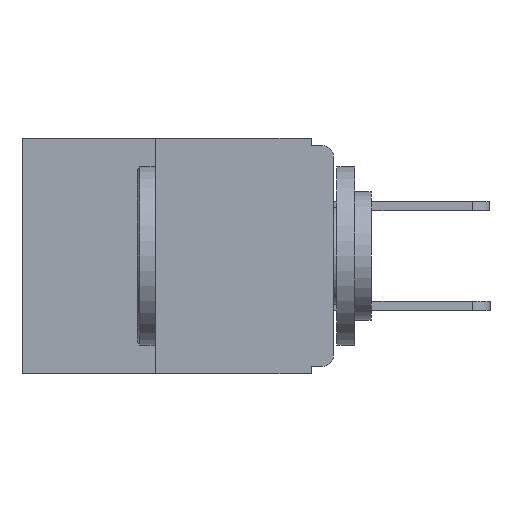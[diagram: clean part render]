
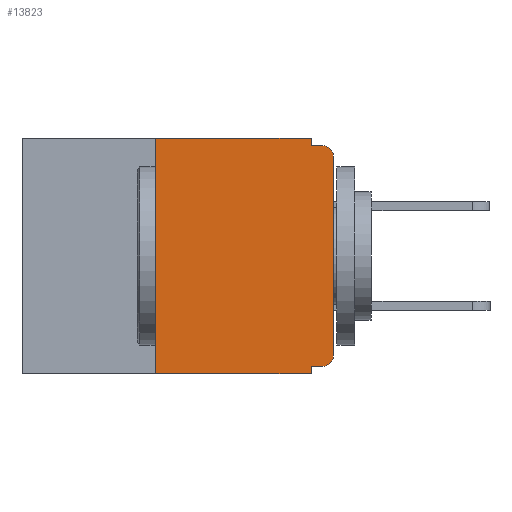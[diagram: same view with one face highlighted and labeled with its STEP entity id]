
A CAD part, left-side view. The second image highlights one B-rep face of the part: STEP entity #13823.
In plain terms, the highlighted planar face has unit normal (-1, 0, 0).
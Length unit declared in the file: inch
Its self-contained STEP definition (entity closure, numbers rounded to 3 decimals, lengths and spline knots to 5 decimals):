
#687 = CARTESIAN_POINT ( 'NONE',  ( 0., 0.031, -0.01 ) ) ;
#865 = EDGE_CURVE ( 'NONE', #14087, #6347, #13229, .T. ) ;
#1225 = VERTEX_POINT ( 'NONE', #6096 ) ;
#1395 = CARTESIAN_POINT ( 'NONE',  ( 0., 0.031, -0.32 ) ) ;
#1573 = EDGE_CURVE ( 'NONE', #8159, #6347, #26481, .T. ) ;
#1597 = VERTEX_POINT ( 'NONE', #7087 ) ;
#1665 = LINE ( 'NONE', #25459, #14906 ) ;
#1934 = DIRECTION ( 'NONE',  ( 0., -1., 0. ) ) ;
#2191 = CARTESIAN_POINT ( 'NONE',  ( 0., 0.437, -0.33 ) ) ;
#4032 = VERTEX_POINT ( 'NONE', #26211 ) ;
#5442 = EDGE_CURVE ( 'NONE', #4032, #1225, #11790, .T. ) ;
#5864 = DIRECTION ( 'NONE',  ( 0., 0., -1. ) ) ;
#5893 = DIRECTION ( 'NONE',  ( -1., 0., 0. ) ) ;
#6096 = CARTESIAN_POINT ( 'NONE',  ( 0., 0., -0.305 ) ) ;
#6266 = CARTESIAN_POINT ( 'NONE',  ( 0., 0.015, -0.305 ) ) ;
#6347 = VERTEX_POINT ( 'NONE', #18890 ) ;
#7087 = CARTESIAN_POINT ( 'NONE',  ( 0., 0.25, 0. ) ) ;
#7190 = VECTOR ( 'NONE', #14193, 39.37008 ) ;
#7679 = LINE ( 'NONE', #24517, #20811 ) ;
#7683 = CARTESIAN_POINT ( 'NONE',  ( 0., 0.015, -0.01 ) ) ;
#8037 = LINE ( 'NONE', #29562, #7190 ) ;
#8159 = VERTEX_POINT ( 'NONE', #1395 ) ;
#8239 = LINE ( 'NONE', #32983, #21327 ) ;
#8891 = EDGE_CURVE ( 'NONE', #22573, #25389, #8239, .T. ) ;
#9546 = VERTEX_POINT ( 'NONE', #32946 ) ;
#9686 = EDGE_CURVE ( 'NONE', #14087, #1597, #18457, .T. ) ;
#9986 = ORIENTED_EDGE ( 'NONE', *, *, #11644, .F. ) ;
#10222 = DIRECTION ( 'NONE',  ( 1., 0., 0. ) ) ;
#10392 = CARTESIAN_POINT ( 'NONE',  ( 0., 0.015, -0.025 ) ) ;
#11644 = EDGE_CURVE ( 'NONE', #4032, #8159, #8037, .T. ) ;
#11784 = EDGE_LOOP ( 'NONE', ( #26076, #27284, #29406, #30085, #30286, #31324, #31380, #19288, #9986, #14053 ) ) ;
#11790 = CIRCLE ( 'NONE', #23067, 0.015 ) ;
#12755 = VECTOR ( 'NONE', #18040, 39.37008 ) ;
#13077 = DIRECTION ( 'NONE',  ( 0., 0., -1. ) ) ;
#13229 = LINE ( 'NONE', #2191, #26107 ) ;
#13823 = ADVANCED_FACE ( 'NONE', ( #24624 ), #18054, .F. ) ;
#14053 = ORIENTED_EDGE ( 'NONE', *, *, #5442, .T. ) ;
#14087 = VERTEX_POINT ( 'NONE', #24075 ) ;
#14193 = DIRECTION ( 'NONE',  ( 0., 1., 0. ) ) ;
#14906 = VECTOR ( 'NONE', #28039, 39.37008 ) ;
#15211 = VECTOR ( 'NONE', #21727, 39.37008 ) ;
#15610 = DIRECTION ( 'NONE',  ( 0., 0., 1. ) ) ;
#15961 = DIRECTION ( 'NONE',  ( 0., -1., 0. ) ) ;
#17026 = CARTESIAN_POINT ( 'NONE',  ( 0., 0.031, -0.33 ) ) ;
#18040 = DIRECTION ( 'NONE',  ( 0., 0., -1. ) ) ;
#18054 = PLANE ( 'NONE',  #32413 ) ;
#18457 = LINE ( 'NONE', #33459, #24453 ) ;
#18890 = CARTESIAN_POINT ( 'NONE',  ( 0., 0.031, -0.33 ) ) ;
#19288 = ORIENTED_EDGE ( 'NONE', *, *, #1573, .F. ) ;
#20329 = VERTEX_POINT ( 'NONE', #30074 ) ;
#20627 = CARTESIAN_POINT ( 'NONE',  ( 0., 0.437, 0. ) ) ;
#20811 = VECTOR ( 'NONE', #27089, 39.37008 ) ;
#21327 = VECTOR ( 'NONE', #1934, 39.37008 ) ;
#21727 = DIRECTION ( 'NONE',  ( 0., 0., 1. ) ) ;
#22573 = VERTEX_POINT ( 'NONE', #687 ) ;
#22860 = EDGE_CURVE ( 'NONE', #1597, #20329, #1665, .T. ) ;
#23067 = AXIS2_PLACEMENT_3D ( 'NONE', #6266, #5893, #5864 ) ;
#24075 = CARTESIAN_POINT ( 'NONE',  ( 0., 0.25, -0.33 ) ) ;
#24267 = CARTESIAN_POINT ( 'NONE',  ( 0., 0., 0. ) ) ;
#24352 = EDGE_CURVE ( 'NONE', #1225, #9546, #28826, .T. ) ;
#24453 = VECTOR ( 'NONE', #15610, 39.37008 ) ;
#24517 = CARTESIAN_POINT ( 'NONE',  ( 0., 0.031, 0. ) ) ;
#24624 = FACE_OUTER_BOUND ( 'NONE', #11784, .T. ) ;
#25389 = VERTEX_POINT ( 'NONE', #7683 ) ;
#25459 = CARTESIAN_POINT ( 'NONE',  ( 0., 0.437, 0. ) ) ;
#25477 = CIRCLE ( 'NONE', #29017, 0.015 ) ;
#26076 = ORIENTED_EDGE ( 'NONE', *, *, #24352, .T. ) ;
#26107 = VECTOR ( 'NONE', #15961, 39.37008 ) ;
#26211 = CARTESIAN_POINT ( 'NONE',  ( 0., 0.015, -0.32 ) ) ;
#26481 = LINE ( 'NONE', #17026, #12755 ) ;
#27089 = DIRECTION ( 'NONE',  ( 0., 0., -1. ) ) ;
#27284 = ORIENTED_EDGE ( 'NONE', *, *, #27345, .T. ) ;
#27345 = EDGE_CURVE ( 'NONE', #9546, #25389, #25477, .T. ) ;
#28039 = DIRECTION ( 'NONE',  ( 0., -1., 0. ) ) ;
#28315 = DIRECTION ( 'NONE',  ( 0., 0., -1. ) ) ;
#28465 = DIRECTION ( 'NONE',  ( -1., 0., 0. ) ) ;
#28826 = LINE ( 'NONE', #24267, #15211 ) ;
#29017 = AXIS2_PLACEMENT_3D ( 'NONE', #10392, #28465, #13077 ) ;
#29406 = ORIENTED_EDGE ( 'NONE', *, *, #8891, .F. ) ;
#29562 = CARTESIAN_POINT ( 'NONE',  ( 0., 0., -0.32 ) ) ;
#30074 = CARTESIAN_POINT ( 'NONE',  ( 0., 0.031, 0. ) ) ;
#30085 = ORIENTED_EDGE ( 'NONE', *, *, #31882, .F. ) ;
#30286 = ORIENTED_EDGE ( 'NONE', *, *, #22860, .F. ) ;
#31324 = ORIENTED_EDGE ( 'NONE', *, *, #9686, .F. ) ;
#31380 = ORIENTED_EDGE ( 'NONE', *, *, #865, .T. ) ;
#31882 = EDGE_CURVE ( 'NONE', #20329, #22573, #7679, .T. ) ;
#32413 = AXIS2_PLACEMENT_3D ( 'NONE', #20627, #10222, #28315 ) ;
#32946 = CARTESIAN_POINT ( 'NONE',  ( 0., 0., -0.025 ) ) ;
#32983 = CARTESIAN_POINT ( 'NONE',  ( 0., 0., -0.01 ) ) ;
#33459 = CARTESIAN_POINT ( 'NONE',  ( 0., 0.25, -0.33 ) ) ;
